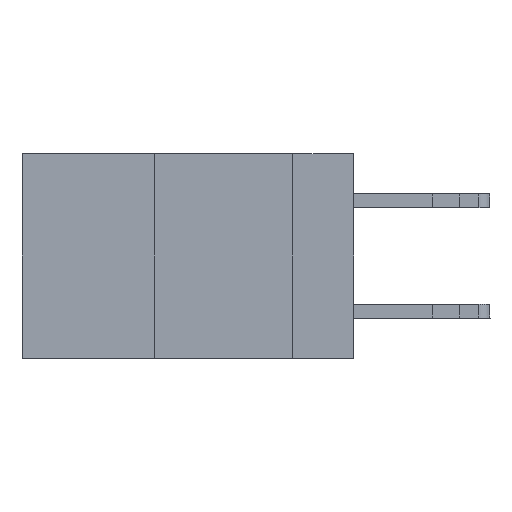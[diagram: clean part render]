
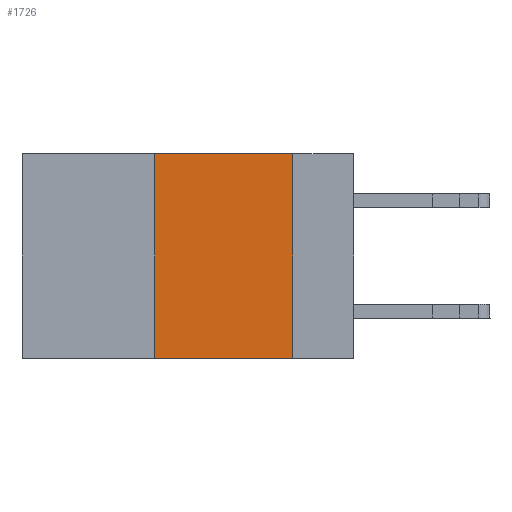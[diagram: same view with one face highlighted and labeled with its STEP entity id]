
A CAD part, left-side view. The second image highlights one B-rep face of the part: STEP entity #1726.
In plain terms, the highlighted planar face has unit normal (-1, 0, 0).
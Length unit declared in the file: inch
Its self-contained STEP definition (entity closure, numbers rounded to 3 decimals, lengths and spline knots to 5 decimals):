
#495 = DIRECTION ( 'NONE',  ( 0., 0., -1. ) ) ;
#1726 = ADVANCED_FACE ( 'NONE', ( #11915 ), #8531, .F. ) ;
#4498 = EDGE_CURVE ( 'NONE', #21741, #5631, #7836, .T. ) ;
#5481 = CARTESIAN_POINT ( 'NONE',  ( 0., 0.11, 0. ) ) ;
#5631 = VERTEX_POINT ( 'NONE', #5839 ) ;
#5839 = CARTESIAN_POINT ( 'NONE',  ( 0., 0.36, 0. ) ) ;
#6901 = ORIENTED_EDGE ( 'NONE', *, *, #19587, .F. ) ;
#7836 = LINE ( 'NONE', #17742, #12364 ) ;
#7892 = AXIS2_PLACEMENT_3D ( 'NONE', #8466, #8435, #8409 ) ;
#8220 = CARTESIAN_POINT ( 'NONE',  ( 0., 0.36, -0.37 ) ) ;
#8385 = LINE ( 'NONE', #9113, #20284 ) ;
#8409 = DIRECTION ( 'NONE',  ( 0., 0., -1. ) ) ;
#8435 = DIRECTION ( 'NONE',  ( 1., 0., 0. ) ) ;
#8466 = CARTESIAN_POINT ( 'NONE',  ( 0., 0.6, 0. ) ) ;
#8531 = PLANE ( 'NONE',  #7892 ) ;
#9005 = EDGE_CURVE ( 'NONE', #18753, #13491, #18689, .T. ) ;
#9113 = CARTESIAN_POINT ( 'NONE',  ( 0., 0.6, -0.37 ) ) ;
#10837 = DIRECTION ( 'NONE',  ( 0., -1., 0. ) ) ;
#11915 = FACE_OUTER_BOUND ( 'NONE', #18895, .T. ) ;
#12076 = VECTOR ( 'NONE', #495, 39.37008 ) ;
#12364 = VECTOR ( 'NONE', #19409, 39.37008 ) ;
#13491 = VERTEX_POINT ( 'NONE', #18767 ) ;
#14131 = DIRECTION ( 'NONE',  ( 0., -1., 0. ) ) ;
#15409 = ORIENTED_EDGE ( 'NONE', *, *, #9005, .F. ) ;
#15936 = ORIENTED_EDGE ( 'NONE', *, *, #4498, .F. ) ;
#16837 = CARTESIAN_POINT ( 'NONE',  ( 0., 0.11, 0. ) ) ;
#16922 = VECTOR ( 'NONE', #14131, 39.37008 ) ;
#17445 = LINE ( 'NONE', #20779, #16922 ) ;
#17742 = CARTESIAN_POINT ( 'NONE',  ( 0., 0.36, 0. ) ) ;
#18689 = LINE ( 'NONE', #5481, #12076 ) ;
#18753 = VERTEX_POINT ( 'NONE', #16837 ) ;
#18767 = CARTESIAN_POINT ( 'NONE',  ( 0., 0.11, -0.37 ) ) ;
#18895 = EDGE_LOOP ( 'NONE', ( #15409, #6901, #15936, #20355 ) ) ;
#19409 = DIRECTION ( 'NONE',  ( 0., 0., 1. ) ) ;
#19587 = EDGE_CURVE ( 'NONE', #5631, #18753, #17445, .T. ) ;
#19635 = EDGE_CURVE ( 'NONE', #21741, #13491, #8385, .T. ) ;
#20284 = VECTOR ( 'NONE', #10837, 39.37008 ) ;
#20355 = ORIENTED_EDGE ( 'NONE', *, *, #19635, .T. ) ;
#20779 = CARTESIAN_POINT ( 'NONE',  ( 0., 0.6, 0. ) ) ;
#21741 = VERTEX_POINT ( 'NONE', #8220 ) ;
